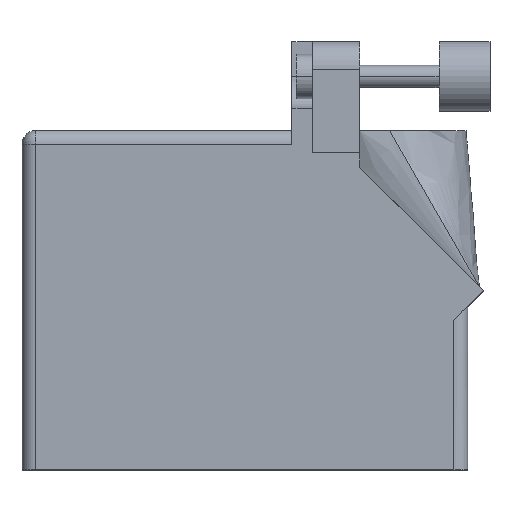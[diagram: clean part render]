
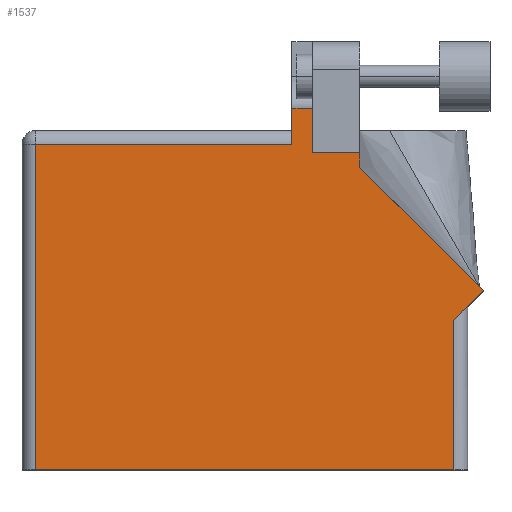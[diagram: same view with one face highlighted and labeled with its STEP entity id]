
A CAD part, top view. The second image highlights one B-rep face of the part: STEP entity #1537.
In plain terms, the highlighted planar face has unit normal (0, 0, 1).
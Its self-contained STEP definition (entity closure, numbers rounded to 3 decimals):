
#7 = EDGE_CURVE ( 'NONE', #646, #902, #1234, .T. ) ;
#12 = DIRECTION ( 'NONE',  ( 0., -1., 0. ) ) ;
#61 = EDGE_CURVE ( 'NONE', #1783, #1503, #2407, .T. ) ;
#115 = ORIENTED_EDGE ( 'NONE', *, *, #256, .T. ) ;
#190 = VERTEX_POINT ( 'NONE', #1768 ) ;
#217 = EDGE_CURVE ( 'NONE', #2471, #1783, #2030, .T. ) ;
#241 = DIRECTION ( 'NONE',  ( 0.707, 0.707, 0. ) ) ;
#245 = CARTESIAN_POINT ( 'NONE',  ( 1.575, 0., 0. ) ) ;
#256 = EDGE_CURVE ( 'NONE', #2394, #2471, #457, .T. ) ;
#333 = DIRECTION ( 'NONE',  ( 0., -1., 0. ) ) ;
#334 = CARTESIAN_POINT ( 'NONE',  ( 38.71, 36.322, 0. ) ) ;
#348 = EDGE_LOOP ( 'NONE', ( #2605, #612, #1294, #823, #1353, #1701, #115, #868, #2202, #2215, #1267 ) ) ;
#378 = CARTESIAN_POINT ( 'NONE',  ( 38.71, 36.322, 0. ) ) ;
#395 = LINE ( 'NONE', #2638, #846 ) ;
#397 = EDGE_CURVE ( 'NONE', #1503, #1001, #410, .T. ) ;
#410 = LINE ( 'NONE', #2705, #2293 ) ;
#424 = LINE ( 'NONE', #1746, #2153 ) ;
#457 = LINE ( 'NONE', #921, #2696 ) ;
#532 = DIRECTION ( 'NONE',  ( -1., 0., 0. ) ) ;
#545 = VERTEX_POINT ( 'NONE', #1747 ) ;
#610 = LINE ( 'NONE', #1489, #1907 ) ;
#612 = ORIENTED_EDGE ( 'NONE', *, *, #2546, .T. ) ;
#626 = DIRECTION ( 'NONE',  ( 0., 1., 0. ) ) ;
#646 = VERTEX_POINT ( 'NONE', #2234 ) ;
#693 = DIRECTION ( 'NONE',  ( 0., 1., 0. ) ) ;
#712 = AXIS2_PLACEMENT_3D ( 'NONE', #954, #2242, #532 ) ;
#730 = EDGE_CURVE ( 'NONE', #1001, #2196, #1253, .T. ) ;
#823 = ORIENTED_EDGE ( 'NONE', *, *, #1124, .T. ) ;
#846 = VECTOR ( 'NONE', #12, 1000. ) ;
#868 = ORIENTED_EDGE ( 'NONE', *, *, #217, .T. ) ;
#902 = VERTEX_POINT ( 'NONE', #245 ) ;
#916 = VECTOR ( 'NONE', #333, 1000. ) ;
#921 = CARTESIAN_POINT ( 'NONE',  ( 49.479, 18.72, 0. ) ) ;
#936 = CARTESIAN_POINT ( 'NONE',  ( 51.054, 18.72, 0. ) ) ;
#948 = VECTOR ( 'NONE', #2352, 1000. ) ;
#954 = CARTESIAN_POINT ( 'NONE',  ( 0., 38.862, 0. ) ) ;
#1001 = VERTEX_POINT ( 'NONE', #334 ) ;
#1120 = LINE ( 'NONE', #2401, #1418 ) ;
#1124 = EDGE_CURVE ( 'NONE', #190, #646, #1120, .T. ) ;
#1147 = EDGE_CURVE ( 'NONE', #2196, #545, #424, .T. ) ;
#1171 = CARTESIAN_POINT ( 'NONE',  ( 33.299, 36.322, 0. ) ) ;
#1200 = VECTOR ( 'NONE', #2146, 1000. ) ;
#1234 = LINE ( 'NONE', #2300, #916 ) ;
#1253 = LINE ( 'NONE', #378, #1470 ) ;
#1256 = LINE ( 'NONE', #2128, #948 ) ;
#1267 = ORIENTED_EDGE ( 'NONE', *, *, #730, .T. ) ;
#1294 = ORIENTED_EDGE ( 'NONE', *, *, #2480, .T. ) ;
#1353 = ORIENTED_EDGE ( 'NONE', *, *, #7, .T. ) ;
#1381 = CARTESIAN_POINT ( 'NONE',  ( 52.85, 20.516, 0. ) ) ;
#1411 = DIRECTION ( 'NONE',  ( 0., 1., 0. ) ) ;
#1418 = VECTOR ( 'NONE', #2179, 1000. ) ;
#1470 = VECTOR ( 'NONE', #1880, 1000. ) ;
#1489 = CARTESIAN_POINT ( 'NONE',  ( 41.701, 41.44, 0. ) ) ;
#1503 = VERTEX_POINT ( 'NONE', #1741 ) ;
#1537 = ADVANCED_FACE ( 'NONE', ( #2721 ), #2048, .F. ) ;
#1665 = CARTESIAN_POINT ( 'NONE',  ( 49.479, 0., 0. ) ) ;
#1701 = ORIENTED_EDGE ( 'NONE', *, *, #1999, .T. ) ;
#1741 = CARTESIAN_POINT ( 'NONE',  ( 38.71, 34.656, 0. ) ) ;
#1746 = CARTESIAN_POINT ( 'NONE',  ( 33.299, 36.322, 0. ) ) ;
#1747 = CARTESIAN_POINT ( 'NONE',  ( 33.299, 41.44, 0. ) ) ;
#1768 = CARTESIAN_POINT ( 'NONE',  ( 30.912, 37.287, 0. ) ) ;
#1783 = VERTEX_POINT ( 'NONE', #1381 ) ;
#1801 = VERTEX_POINT ( 'NONE', #2269 ) ;
#1880 = DIRECTION ( 'NONE',  ( -1., 0., 0. ) ) ;
#1907 = VECTOR ( 'NONE', #2151, 1000. ) ;
#1999 = EDGE_CURVE ( 'NONE', #902, #2394, #1256, .T. ) ;
#2030 = LINE ( 'NONE', #936, #2383 ) ;
#2048 = PLANE ( 'NONE',  #712 ) ;
#2128 = CARTESIAN_POINT ( 'NONE',  ( 0., 0., 0. ) ) ;
#2146 = DIRECTION ( 'NONE',  ( -0.707, 0.707, 0. ) ) ;
#2151 = DIRECTION ( 'NONE',  ( -1., 0., 0. ) ) ;
#2153 = VECTOR ( 'NONE', #626, 1000. ) ;
#2179 = DIRECTION ( 'NONE',  ( -1., 0., 0. ) ) ;
#2196 = VERTEX_POINT ( 'NONE', #1171 ) ;
#2202 = ORIENTED_EDGE ( 'NONE', *, *, #61, .T. ) ;
#2215 = ORIENTED_EDGE ( 'NONE', *, *, #397, .T. ) ;
#2234 = CARTESIAN_POINT ( 'NONE',  ( 1.575, 37.287, 0. ) ) ;
#2242 = DIRECTION ( 'NONE',  ( 0., 0., -1. ) ) ;
#2269 = CARTESIAN_POINT ( 'NONE',  ( 30.912, 41.44, 0. ) ) ;
#2293 = VECTOR ( 'NONE', #1411, 1000. ) ;
#2300 = CARTESIAN_POINT ( 'NONE',  ( 1.575, 0., 0. ) ) ;
#2352 = DIRECTION ( 'NONE',  ( 1., 0., 0. ) ) ;
#2383 = VECTOR ( 'NONE', #241, 1000. ) ;
#2394 = VERTEX_POINT ( 'NONE', #1665 ) ;
#2401 = CARTESIAN_POINT ( 'NONE',  ( 0., 37.287, 0. ) ) ;
#2407 = LINE ( 'NONE', #2841, #1200 ) ;
#2471 = VERTEX_POINT ( 'NONE', #2802 ) ;
#2480 = EDGE_CURVE ( 'NONE', #1801, #190, #395, .T. ) ;
#2546 = EDGE_CURVE ( 'NONE', #545, #1801, #610, .T. ) ;
#2605 = ORIENTED_EDGE ( 'NONE', *, *, #1147, .T. ) ;
#2638 = CARTESIAN_POINT ( 'NONE',  ( 30.912, 38.862, 0. ) ) ;
#2696 = VECTOR ( 'NONE', #693, 1000. ) ;
#2705 = CARTESIAN_POINT ( 'NONE',  ( 38.71, 34.656, 0. ) ) ;
#2721 = FACE_OUTER_BOUND ( 'NONE', #348, .T. ) ;
#2802 = CARTESIAN_POINT ( 'NONE',  ( 49.479, 17.145, 0. ) ) ;
#2841 = CARTESIAN_POINT ( 'NONE',  ( 52.85, 20.516, 0. ) ) ;
